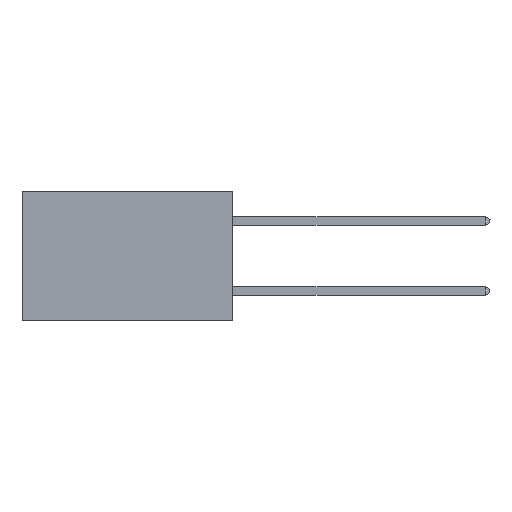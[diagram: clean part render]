
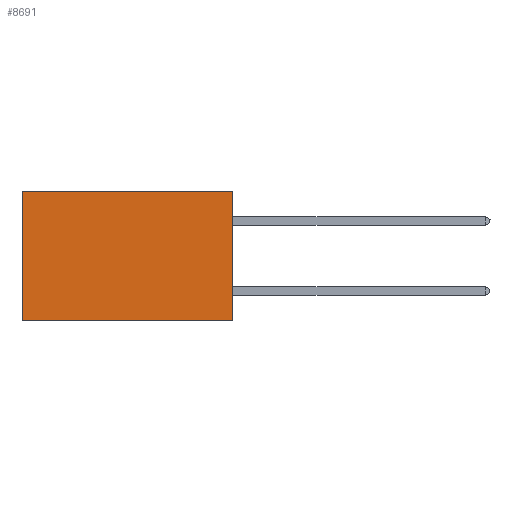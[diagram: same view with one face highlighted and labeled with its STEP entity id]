
A CAD part, left-side view. The second image highlights one B-rep face of the part: STEP entity #8691.
In plain terms, the highlighted planar face has unit normal (-1, 0, 0).
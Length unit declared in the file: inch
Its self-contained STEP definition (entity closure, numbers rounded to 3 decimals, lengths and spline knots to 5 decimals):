
#530 = ORIENTED_EDGE ( 'NONE', *, *, #26506, .F. ) ;
#592 = DIRECTION ( 'NONE',  ( 0., 0., -1. ) ) ;
#596 = LINE ( 'NONE', #7788, #6573 ) ;
#1052 = VECTOR ( 'NONE', #16097, 39.37008 ) ;
#1327 = AXIS2_PLACEMENT_3D ( 'NONE', #2539, #11090, #592 ) ;
#2164 = DIRECTION ( 'NONE',  ( 0., 0., -1. ) ) ;
#2255 = CARTESIAN_POINT ( 'NONE',  ( 0.2875, 0.6, 0. ) ) ;
#2539 = CARTESIAN_POINT ( 'NONE',  ( 0.2875, 0., 0. ) ) ;
#3446 = DIRECTION ( 'NONE',  ( 0., 0., -1. ) ) ;
#3565 = CARTESIAN_POINT ( 'NONE',  ( 0.2875, 0., 0. ) ) ;
#3706 = VERTEX_POINT ( 'NONE', #25360 ) ;
#4054 = VECTOR ( 'NONE', #2164, 39.37008 ) ;
#4871 = VERTEX_POINT ( 'NONE', #20914 ) ;
#5283 = EDGE_LOOP ( 'NONE', ( #8580, #530, #13208, #16771 ) ) ;
#6573 = VECTOR ( 'NONE', #8075, 39.37008 ) ;
#7788 = CARTESIAN_POINT ( 'NONE',  ( 0.2875, 0., 0. ) ) ;
#8075 = DIRECTION ( 'NONE',  ( 0., 1., 0. ) ) ;
#8580 = ORIENTED_EDGE ( 'NONE', *, *, #26278, .T. ) ;
#8691 = ADVANCED_FACE ( 'NONE', ( #23763 ), #21564, .F. ) ;
#9434 = CARTESIAN_POINT ( 'NONE',  ( 0.2875, 0.6, -0.37 ) ) ;
#11090 = DIRECTION ( 'NONE',  ( 1., 0., 0. ) ) ;
#12382 = LINE ( 'NONE', #2255, #4054 ) ;
#12418 = EDGE_CURVE ( 'NONE', #21215, #3706, #24953, .T. ) ;
#13208 = ORIENTED_EDGE ( 'NONE', *, *, #12418, .F. ) ;
#13655 = VECTOR ( 'NONE', #3446, 39.37008 ) ;
#14461 = EDGE_CURVE ( 'NONE', #21215, #4871, #596, .T. ) ;
#16097 = DIRECTION ( 'NONE',  ( 0., 1., 0. ) ) ;
#16222 = CARTESIAN_POINT ( 'NONE',  ( 0.2875, 0., 0. ) ) ;
#16771 = ORIENTED_EDGE ( 'NONE', *, *, #14461, .T. ) ;
#18222 = VERTEX_POINT ( 'NONE', #9434 ) ;
#20914 = CARTESIAN_POINT ( 'NONE',  ( 0.2875, 0.6, 0. ) ) ;
#21215 = VERTEX_POINT ( 'NONE', #3565 ) ;
#21564 = PLANE ( 'NONE',  #1327 ) ;
#23763 = FACE_OUTER_BOUND ( 'NONE', #5283, .T. ) ;
#24370 = CARTESIAN_POINT ( 'NONE',  ( 0.2875, 0., -0.37 ) ) ;
#24953 = LINE ( 'NONE', #16222, #13655 ) ;
#25360 = CARTESIAN_POINT ( 'NONE',  ( 0.2875, 0., -0.37 ) ) ;
#26278 = EDGE_CURVE ( 'NONE', #4871, #18222, #12382, .T. ) ;
#26312 = LINE ( 'NONE', #24370, #1052 ) ;
#26506 = EDGE_CURVE ( 'NONE', #3706, #18222, #26312, .T. ) ;
